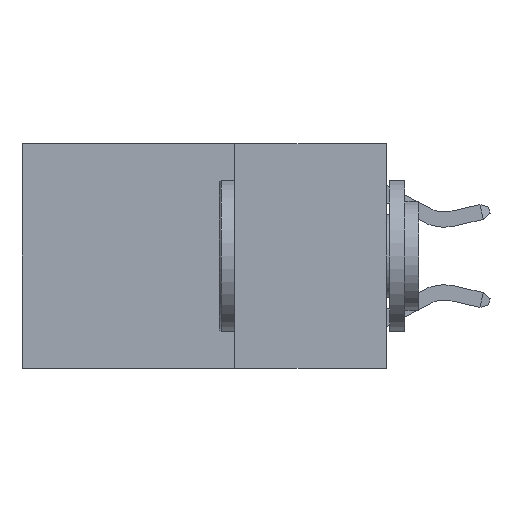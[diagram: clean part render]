
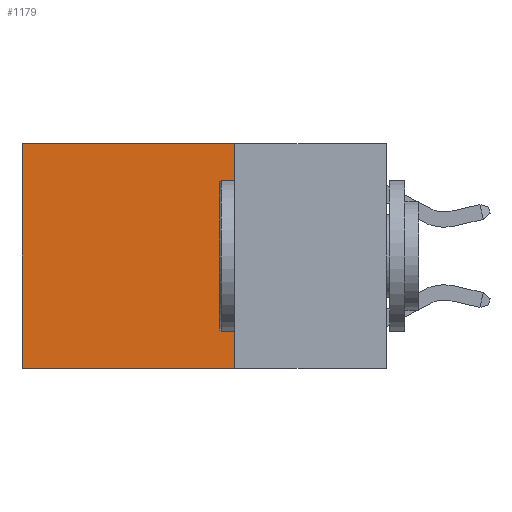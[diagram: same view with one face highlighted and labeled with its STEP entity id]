
A CAD part, left-side view. The second image highlights one B-rep face of the part: STEP entity #1179.
In plain terms, the highlighted planar face has unit normal (-1, 0, 0).
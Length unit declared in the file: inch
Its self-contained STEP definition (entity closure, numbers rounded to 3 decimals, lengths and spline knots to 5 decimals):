
#1179 = ADVANCED_FACE ( 'NONE', ( #14834 ), #20559, .F. ) ;
#1191 = EDGE_LOOP ( 'NONE', ( #15004, #18930, #22724, #17534 ) ) ;
#1441 = VECTOR ( 'NONE', #22045, 39.37008 ) ;
#3911 = VECTOR ( 'NONE', #20659, 39.37008 ) ;
#5371 = EDGE_CURVE ( 'NONE', #16841, #8150, #15501, .T. ) ;
#5511 = DIRECTION ( 'NONE',  ( 1., 0., 0. ) ) ;
#5592 = EDGE_CURVE ( 'NONE', #9566, #12931, #12459, .T. ) ;
#5980 = CARTESIAN_POINT ( 'NONE',  ( 0.2625, 0.25, 0. ) ) ;
#7762 = CARTESIAN_POINT ( 'NONE',  ( 0.2625, 0.6, -0.37 ) ) ;
#8150 = VERTEX_POINT ( 'NONE', #19602 ) ;
#9372 = VECTOR ( 'NONE', #11255, 39.37008 ) ;
#9566 = VERTEX_POINT ( 'NONE', #15074 ) ;
#10198 = AXIS2_PLACEMENT_3D ( 'NONE', #20193, #5511, #20674 ) ;
#11255 = DIRECTION ( 'NONE',  ( 0., 1., 0. ) ) ;
#12459 = LINE ( 'NONE', #14472, #1441 ) ;
#12931 = VERTEX_POINT ( 'NONE', #7762 ) ;
#13060 = CARTESIAN_POINT ( 'NONE',  ( 0.2625, 0.6, 0. ) ) ;
#13099 = LINE ( 'NONE', #5980, #19117 ) ;
#13214 = EDGE_CURVE ( 'NONE', #8150, #12931, #21019, .T. ) ;
#14472 = CARTESIAN_POINT ( 'NONE',  ( 0.2625, 0.25, -0.37 ) ) ;
#14834 = FACE_OUTER_BOUND ( 'NONE', #1191, .T. ) ;
#15004 = ORIENTED_EDGE ( 'NONE', *, *, #13214, .T. ) ;
#15074 = CARTESIAN_POINT ( 'NONE',  ( 0.2625, 0.25, -0.37 ) ) ;
#15501 = LINE ( 'NONE', #18738, #9372 ) ;
#16841 = VERTEX_POINT ( 'NONE', #18985 ) ;
#17291 = EDGE_CURVE ( 'NONE', #16841, #9566, #13099, .T. ) ;
#17534 = ORIENTED_EDGE ( 'NONE', *, *, #5371, .T. ) ;
#18738 = CARTESIAN_POINT ( 'NONE',  ( 0.2625, 0.25, 0. ) ) ;
#18930 = ORIENTED_EDGE ( 'NONE', *, *, #5592, .F. ) ;
#18985 = CARTESIAN_POINT ( 'NONE',  ( 0.2625, 0.25, 0. ) ) ;
#19117 = VECTOR ( 'NONE', #23057, 39.37008 ) ;
#19602 = CARTESIAN_POINT ( 'NONE',  ( 0.2625, 0.6, 0. ) ) ;
#20193 = CARTESIAN_POINT ( 'NONE',  ( 0.2625, 0.25, 0. ) ) ;
#20559 = PLANE ( 'NONE',  #10198 ) ;
#20659 = DIRECTION ( 'NONE',  ( 0., 0., -1. ) ) ;
#20674 = DIRECTION ( 'NONE',  ( 0., 0., -1. ) ) ;
#21019 = LINE ( 'NONE', #13060, #3911 ) ;
#22045 = DIRECTION ( 'NONE',  ( 0., 1., 0. ) ) ;
#22724 = ORIENTED_EDGE ( 'NONE', *, *, #17291, .F. ) ;
#23057 = DIRECTION ( 'NONE',  ( 0., 0., -1. ) ) ;
